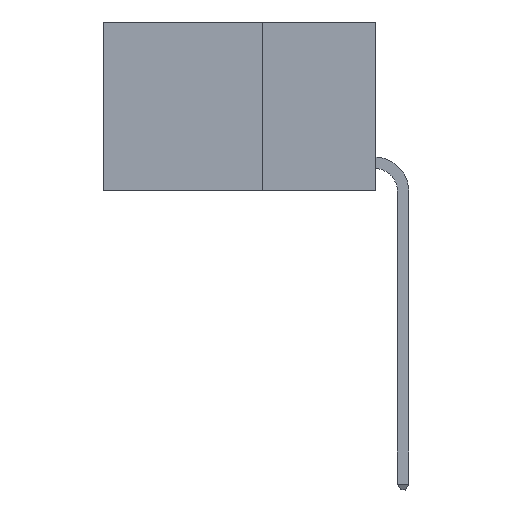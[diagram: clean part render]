
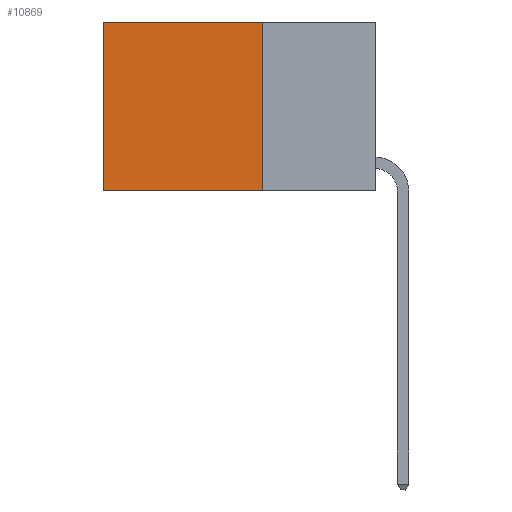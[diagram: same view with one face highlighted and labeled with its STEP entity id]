
A CAD part, left-side view. The second image highlights one B-rep face of the part: STEP entity #10869.
In plain terms, the highlighted planar face has unit normal (-1, 0, 0).
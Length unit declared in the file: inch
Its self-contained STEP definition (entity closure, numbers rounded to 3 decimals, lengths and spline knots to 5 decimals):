
#365 = CARTESIAN_POINT ( 'NONE',  ( 0.2625, 0.25, 0. ) ) ;
#676 = DIRECTION ( 'NONE',  ( 0., 0., -1. ) ) ;
#813 = DIRECTION ( 'NONE',  ( 0., 0., -1. ) ) ;
#815 = CARTESIAN_POINT ( 'NONE',  ( 0.2625, 0.6, 0. ) ) ;
#1044 = VERTEX_POINT ( 'NONE', #9198 ) ;
#1584 = VECTOR ( 'NONE', #5091, 39.37008 ) ;
#1612 = CARTESIAN_POINT ( 'NONE',  ( 0.2625, 0.25, 0. ) ) ;
#1822 = ORIENTED_EDGE ( 'NONE', *, *, #11665, .F. ) ;
#3042 = VECTOR ( 'NONE', #5882, 39.37008 ) ;
#3433 = VERTEX_POINT ( 'NONE', #5429 ) ;
#3685 = FACE_OUTER_BOUND ( 'NONE', #6017, .T. ) ;
#3948 = VERTEX_POINT ( 'NONE', #1612 ) ;
#4010 = EDGE_CURVE ( 'NONE', #1044, #4212, #7437, .T. ) ;
#4212 = VERTEX_POINT ( 'NONE', #8469 ) ;
#4356 = ORIENTED_EDGE ( 'NONE', *, *, #6209, .F. ) ;
#4966 = EDGE_CURVE ( 'NONE', #3948, #1044, #6592, .T. ) ;
#5091 = DIRECTION ( 'NONE',  ( 0., 1., 0. ) ) ;
#5406 = PLANE ( 'NONE',  #8513 ) ;
#5429 = CARTESIAN_POINT ( 'NONE',  ( 0.2625, 0.25, -0.37 ) ) ;
#5544 = LINE ( 'NONE', #8636, #3042 ) ;
#5795 = ORIENTED_EDGE ( 'NONE', *, *, #4966, .T. ) ;
#5832 = VECTOR ( 'NONE', #7976, 39.37008 ) ;
#5882 = DIRECTION ( 'NONE',  ( 0., 0., -1. ) ) ;
#6017 = EDGE_LOOP ( 'NONE', ( #8869, #1822, #4356, #5795 ) ) ;
#6209 = EDGE_CURVE ( 'NONE', #3948, #3433, #5544, .T. ) ;
#6326 = DIRECTION ( 'NONE',  ( 1., 0., 0. ) ) ;
#6592 = LINE ( 'NONE', #365, #1584 ) ;
#7150 = VECTOR ( 'NONE', #813, 39.37008 ) ;
#7437 = LINE ( 'NONE', #815, #7150 ) ;
#7976 = DIRECTION ( 'NONE',  ( 0., 1., 0. ) ) ;
#8469 = CARTESIAN_POINT ( 'NONE',  ( 0.2625, 0.6, -0.37 ) ) ;
#8513 = AXIS2_PLACEMENT_3D ( 'NONE', #11824, #6326, #676 ) ;
#8636 = CARTESIAN_POINT ( 'NONE',  ( 0.2625, 0.25, 0. ) ) ;
#8869 = ORIENTED_EDGE ( 'NONE', *, *, #4010, .T. ) ;
#9198 = CARTESIAN_POINT ( 'NONE',  ( 0.2625, 0.6, 0. ) ) ;
#10712 = LINE ( 'NONE', #11161, #5832 ) ;
#10869 = ADVANCED_FACE ( 'NONE', ( #3685 ), #5406, .F. ) ;
#11161 = CARTESIAN_POINT ( 'NONE',  ( 0.2625, 0.25, -0.37 ) ) ;
#11665 = EDGE_CURVE ( 'NONE', #3433, #4212, #10712, .T. ) ;
#11824 = CARTESIAN_POINT ( 'NONE',  ( 0.2625, 0.25, 0. ) ) ;
